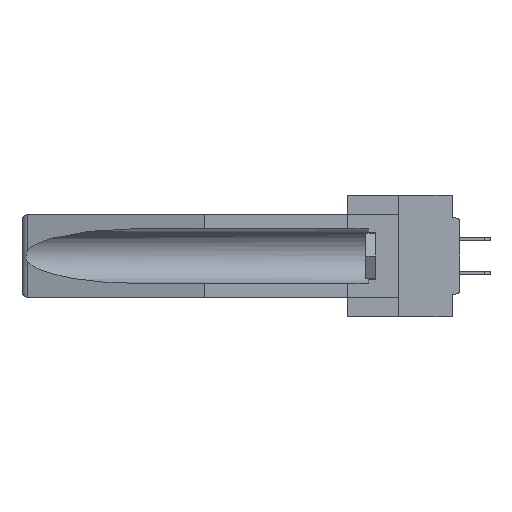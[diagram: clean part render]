
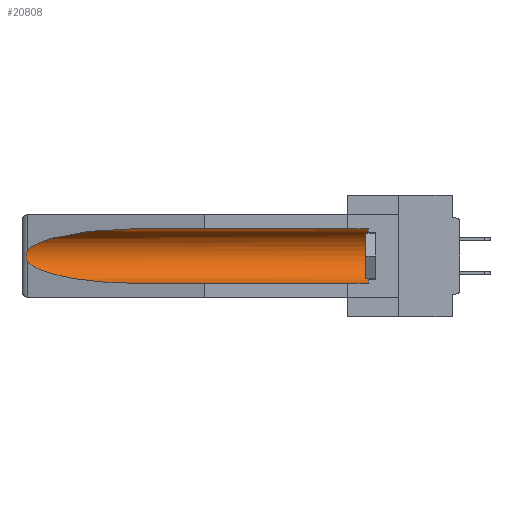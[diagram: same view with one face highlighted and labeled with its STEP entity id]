
A CAD part, left-side view. The second image highlights one B-rep face of the part: STEP entity #20808.
In plain terms, the highlighted cylindrical face has radius 2.857 mm (diameter 5.715 mm), a partial arc.
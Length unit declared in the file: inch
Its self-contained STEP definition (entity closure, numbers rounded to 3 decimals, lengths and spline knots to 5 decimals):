
#105 = FACE_OUTER_BOUND ( 'NONE', #959, .T. ) ;
#219 = VERTEX_POINT ( 'NONE', #17104 ) ;
#821 = EDGE_CURVE ( 'NONE', #19566, #20630, #21168, .T. ) ;
#959 = EDGE_LOOP ( 'NONE', ( #23427, #25879, #3585, #22274, #6891, #15465 ) ) ;
#2008 = CARTESIAN_POINT ( 'NONE',  ( 0.21114, 1.30732, -0.284 ) ) ;
#3011 = EDGE_CURVE ( 'NONE', #19566, #219, #22294, .T. ) ;
#3196 = CARTESIAN_POINT ( 'NONE',  ( 0.2673, 1.53269, -0.17917 ) ) ;
#3328 = CARTESIAN_POINT ( 'NONE',  ( 0.155, 0.126, -0.059 ) ) ;
#3585 = ORIENTED_EDGE ( 'NONE', *, *, #23696, .T. ) ;
#6205 = CARTESIAN_POINT ( 'NONE',  ( 0.2673, 1.5327, -0.16383 ) ) ;
#6891 = ORIENTED_EDGE ( 'NONE', *, *, #821, .T. ) ;
#7347 = CARTESIAN_POINT ( 'NONE',  ( 0.25451, 1.48313, -0.24835 ) ) ;
#9901 = AXIS2_PLACEMENT_3D ( 'NONE', #31034, #31272, #17930 ) ;
#10397 = CARTESIAN_POINT ( 'NONE',  ( 0.26537, 1.52718, -0.14972 ) ) ;
#11179 = CARTESIAN_POINT ( 'NONE',  ( 0.26537, 1.52718, -0.14972 ) ) ;
#11401 = CARTESIAN_POINT ( 'NONE',  ( 0.155, 0.126, -0.284 ) ) ;
#13951 = CARTESIAN_POINT ( 'NONE',  ( 0.26597, 1.52961, -0.15275 ) ) ;
#14952 = EDGE_CURVE ( 'NONE', #25553, #28535, #28637, .T. ) ;
#15184 = CARTESIAN_POINT ( 'NONE',  ( 0.26537, 1.52718, -0.19328 ) ) ;
#15238 = CARTESIAN_POINT ( 'NONE',  ( 0.155, -0.30754, -0.284 ) ) ;
#15465 = ORIENTED_EDGE ( 'NONE', *, *, #30266, .T. ) ;
#16352 = LINE ( 'NONE', #19721, #32962 ) ;
#16399 = CARTESIAN_POINT ( 'NONE',  ( 0.26537, 1.52718, -0.19328 ) ) ;
#16665 = DIRECTION ( 'NONE',  ( 0., 1., 0. ) ) ;
#17104 = CARTESIAN_POINT ( 'NONE',  ( 0.155, 1.07973, -0.284 ) ) ;
#17568 = VERTEX_POINT ( 'NONE', #28714 ) ;
#17930 = DIRECTION ( 'NONE',  ( 0., 0., 1. ) ) ;
#18194 = CARTESIAN_POINT ( 'NONE',  ( 0.155, 1.07973, -0.059 ) ) ;
#19068 = CARTESIAN_POINT ( 'NONE',  ( 0.26655, 1.53094, -0.18657 ) ) ;
#19321 = CARTESIAN_POINT ( 'NONE',  ( 0.26597, 1.5296, -0.19026 ) ) ;
#19566 = VERTEX_POINT ( 'NONE', #11401 ) ;
#19721 = CARTESIAN_POINT ( 'NONE',  ( 0.155, -0.30754, -0.059 ) ) ;
#20630 = VERTEX_POINT ( 'NONE', #3328 ) ;
#20808 = ADVANCED_FACE ( 'NONE', ( #105 ), #29503, .F. ) ;
#21168 = CIRCLE ( 'NONE', #9901, 0.1125 ) ;
#21354 = AXIS2_PLACEMENT_3D ( 'NONE', #26212, #28953, #34223 ) ;
#22274 = ORIENTED_EDGE ( 'NONE', *, *, #3011, .F. ) ;
#22294 = LINE ( 'NONE', #15238, #27255 ) ;
#22543 = DIRECTION ( 'NONE',  ( 0., 1., 0. ) ) ;
#23427 = ORIENTED_EDGE ( 'NONE', *, *, #31753, .T. ) ;
#23696 = EDGE_CURVE ( 'NONE', #28535, #219, #33755, .T. ) ;
#23943 =( BOUNDED_CURVE ( )  B_SPLINE_CURVE ( 3, ( #18194, #26211, #26332, #10397 ),
 .UNSPECIFIED., .F., .F. ) 
 B_SPLINE_CURVE_WITH_KNOTS ( ( 4, 4 ),
 ( 4.71239, 6.08839 ),
 .UNSPECIFIED. ) 
 CURVE ( )  GEOMETRIC_REPRESENTATION_ITEM ( )  RATIONAL_B_SPLINE_CURVE ( ( 1., 0.848, 0.848, 1. ) ) 
 REPRESENTATION_ITEM ( '' )  );
#25465 = CARTESIAN_POINT ( 'NONE',  ( 0.26537, 1.52718, -0.19328 ) ) ;
#25553 = VERTEX_POINT ( 'NONE', #31747 ) ;
#25879 = ORIENTED_EDGE ( 'NONE', *, *, #14952, .T. ) ;
#26211 = CARTESIAN_POINT ( 'NONE',  ( 0.21114, 1.30732, -0.059 ) ) ;
#26212 = CARTESIAN_POINT ( 'NONE',  ( 0.155, -0.30754, -0.1715 ) ) ;
#26332 = CARTESIAN_POINT ( 'NONE',  ( 0.25451, 1.48313, -0.09465 ) ) ;
#27255 = VECTOR ( 'NONE', #22543, 39.37008 ) ;
#28220 = CARTESIAN_POINT ( 'NONE',  ( 0.155, 1.07973, -0.284 ) ) ;
#28535 = VERTEX_POINT ( 'NONE', #25465 ) ;
#28637 = B_SPLINE_CURVE_WITH_KNOTS ( 'NONE', 3,
 ( #11179, #13951, #32648, #6205, #32532, #30065, #3196, #19068, #19321, #16399 ),
 .UNSPECIFIED., .F., .F.,
 ( 4, 2, 2, 2, 4 ),
 ( 0., 0.00029, 0.00058, 0.00087, 0.00117 ),
 .UNSPECIFIED. ) ;
#28714 = CARTESIAN_POINT ( 'NONE',  ( 0.155, 1.07973, -0.059 ) ) ;
#28953 = DIRECTION ( 'NONE',  ( 0., 1., 0. ) ) ;
#29503 = CYLINDRICAL_SURFACE ( 'NONE', #21354, 0.1125 ) ;
#30065 = CARTESIAN_POINT ( 'NONE',  ( 0.2675, 1.53308, -0.17534 ) ) ;
#30266 = EDGE_CURVE ( 'NONE', #20630, #17568, #16352, .T. ) ;
#31034 = CARTESIAN_POINT ( 'NONE',  ( 0.155, 0.126, -0.1715 ) ) ;
#31272 = DIRECTION ( 'NONE',  ( 0., -1., 0. ) ) ;
#31747 = CARTESIAN_POINT ( 'NONE',  ( 0.26537, 1.52718, -0.14972 ) ) ;
#31753 = EDGE_CURVE ( 'NONE', #17568, #25553, #23943, .T. ) ;
#32532 = CARTESIAN_POINT ( 'NONE',  ( 0.2675, 1.53308, -0.16763 ) ) ;
#32648 = CARTESIAN_POINT ( 'NONE',  ( 0.26654, 1.53092, -0.15636 ) ) ;
#32962 = VECTOR ( 'NONE', #16665, 39.37008 ) ;
#33755 =( BOUNDED_CURVE ( )  B_SPLINE_CURVE ( 3, ( #15184, #7347, #2008, #28220 ),
 .UNSPECIFIED., .F., .F. ) 
 B_SPLINE_CURVE_WITH_KNOTS ( ( 4, 4 ),
 ( 0.1948, 1.5708 ),
 .UNSPECIFIED. ) 
 CURVE ( )  GEOMETRIC_REPRESENTATION_ITEM ( )  RATIONAL_B_SPLINE_CURVE ( ( 1., 0.848, 0.848, 1. ) ) 
 REPRESENTATION_ITEM ( '' )  );
#34223 = DIRECTION ( 'NONE',  ( 0., 0., 1. ) ) ;
